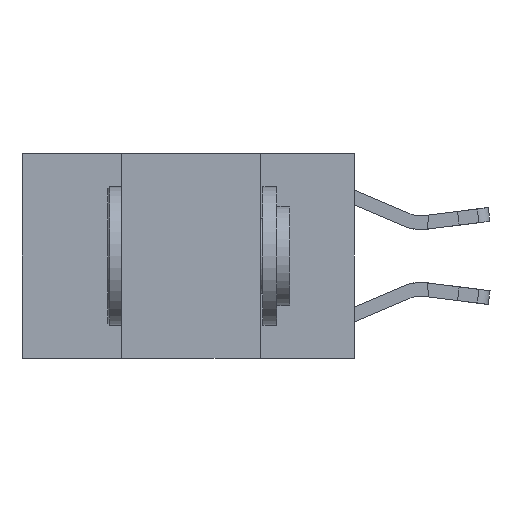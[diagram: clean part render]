
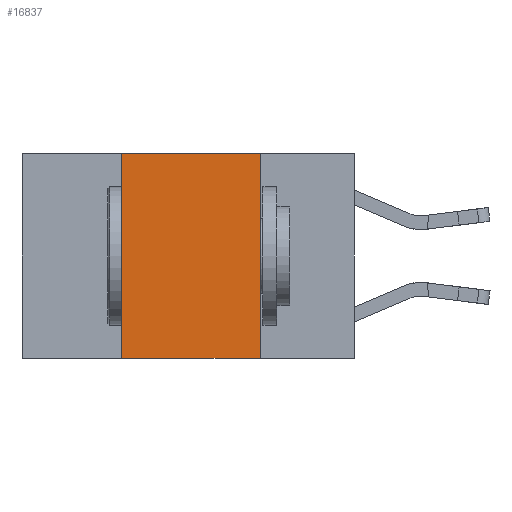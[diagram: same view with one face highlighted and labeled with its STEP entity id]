
A CAD part, left-side view. The second image highlights one B-rep face of the part: STEP entity #16837.
In plain terms, the highlighted planar face has unit normal (-1, 0, 0).
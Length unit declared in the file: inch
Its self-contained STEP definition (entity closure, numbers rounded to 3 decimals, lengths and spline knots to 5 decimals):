
#3649 = EDGE_CURVE ( 'NONE', #4200, #5050, #19745, .T. ) ;
#3879 = CARTESIAN_POINT ( 'NONE',  ( 0., 0.42, 0. ) ) ;
#3947 = CARTESIAN_POINT ( 'NONE',  ( 0., 0.17, 0. ) ) ;
#4120 = CARTESIAN_POINT ( 'NONE',  ( 0., 0.6, 0. ) ) ;
#4200 = VERTEX_POINT ( 'NONE', #5134 ) ;
#4444 = CARTESIAN_POINT ( 'NONE',  ( 0., 0.6, 0. ) ) ;
#5050 = VERTEX_POINT ( 'NONE', #3879 ) ;
#5134 = CARTESIAN_POINT ( 'NONE',  ( 0., 0.42, -0.37 ) ) ;
#5706 = DIRECTION ( 'NONE',  ( 0., -1., 0. ) ) ;
#6022 = DIRECTION ( 'NONE',  ( 0., 0., -1. ) ) ;
#6131 = VECTOR ( 'NONE', #16797, 39.37008 ) ;
#6160 = LINE ( 'NONE', #17466, #18226 ) ;
#6180 = LINE ( 'NONE', #4120, #9852 ) ;
#6420 = VERTEX_POINT ( 'NONE', #3947 ) ;
#7116 = EDGE_CURVE ( 'NONE', #6420, #10831, #10302, .T. ) ;
#7989 = DIRECTION ( 'NONE',  ( 0., -1., 0. ) ) ;
#8122 = ORIENTED_EDGE ( 'NONE', *, *, #7116, .F. ) ;
#9562 = AXIS2_PLACEMENT_3D ( 'NONE', #4444, #15461, #6022 ) ;
#9852 = VECTOR ( 'NONE', #5706, 39.37008 ) ;
#10302 = LINE ( 'NONE', #13617, #6131 ) ;
#10309 = ORIENTED_EDGE ( 'NONE', *, *, #13792, .F. ) ;
#10831 = VERTEX_POINT ( 'NONE', #20126 ) ;
#10881 = ORIENTED_EDGE ( 'NONE', *, *, #3649, .F. ) ;
#11317 = CARTESIAN_POINT ( 'NONE',  ( 0., 0.42, 0. ) ) ;
#12278 = PLANE ( 'NONE',  #9562 ) ;
#12912 = DIRECTION ( 'NONE',  ( 0., 0., 1. ) ) ;
#13617 = CARTESIAN_POINT ( 'NONE',  ( 0., 0.17, 0. ) ) ;
#13792 = EDGE_CURVE ( 'NONE', #5050, #6420, #6180, .T. ) ;
#14123 = EDGE_CURVE ( 'NONE', #4200, #10831, #6160, .T. ) ;
#14733 = ORIENTED_EDGE ( 'NONE', *, *, #14123, .T. ) ;
#14923 = EDGE_LOOP ( 'NONE', ( #8122, #10309, #10881, #14733 ) ) ;
#15461 = DIRECTION ( 'NONE',  ( 1., 0., 0. ) ) ;
#15616 = VECTOR ( 'NONE', #12912, 39.37008 ) ;
#16758 = FACE_OUTER_BOUND ( 'NONE', #14923, .T. ) ;
#16797 = DIRECTION ( 'NONE',  ( 0., 0., -1. ) ) ;
#16837 = ADVANCED_FACE ( 'NONE', ( #16758 ), #12278, .F. ) ;
#17466 = CARTESIAN_POINT ( 'NONE',  ( 0., 0.6, -0.37 ) ) ;
#18226 = VECTOR ( 'NONE', #7989, 39.37008 ) ;
#19745 = LINE ( 'NONE', #11317, #15616 ) ;
#20126 = CARTESIAN_POINT ( 'NONE',  ( 0., 0.17, -0.37 ) ) ;
